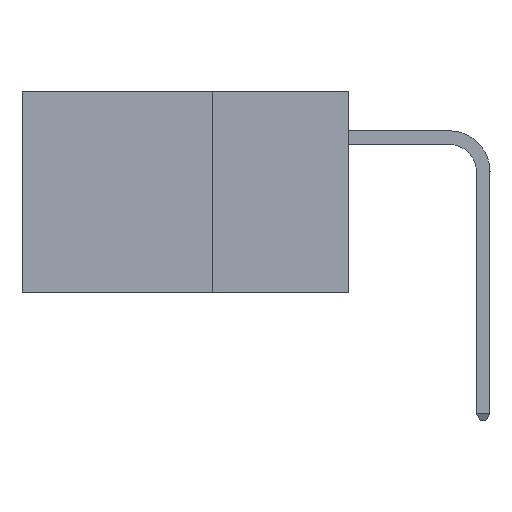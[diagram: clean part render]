
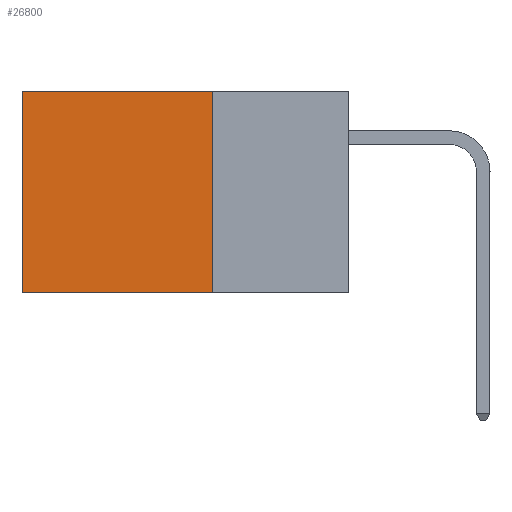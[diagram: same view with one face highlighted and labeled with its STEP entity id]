
A CAD part, left-side view. The second image highlights one B-rep face of the part: STEP entity #26800.
In plain terms, the highlighted planar face has unit normal (-1, 0, 0).
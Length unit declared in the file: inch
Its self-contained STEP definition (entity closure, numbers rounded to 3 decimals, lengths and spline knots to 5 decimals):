
#557 = AXIS2_PLACEMENT_3D ( 'NONE', #37824, #31231, #34038 ) ;
#2293 = VECTOR ( 'NONE', #39726, 39.37008 ) ;
#2990 = DIRECTION ( 'NONE',  ( 0., 1., 0. ) ) ;
#7943 = CARTESIAN_POINT ( 'NONE',  ( 0.2875, 0.25, -0.37 ) ) ;
#8426 = VERTEX_POINT ( 'NONE', #20932 ) ;
#8679 = ORIENTED_EDGE ( 'NONE', *, *, #34176, .F. ) ;
#10671 = LINE ( 'NONE', #29616, #2293 ) ;
#12852 = ORIENTED_EDGE ( 'NONE', *, *, #26646, .T. ) ;
#12959 = CARTESIAN_POINT ( 'NONE',  ( 0.2875, 0.25, -0.37 ) ) ;
#13075 = CARTESIAN_POINT ( 'NONE',  ( 0.2875, 0.6, 0. ) ) ;
#13395 = EDGE_CURVE ( 'NONE', #13584, #17187, #36282, .T. ) ;
#13584 = VERTEX_POINT ( 'NONE', #7943 ) ;
#17187 = VERTEX_POINT ( 'NONE', #40276 ) ;
#18881 = VECTOR ( 'NONE', #23900, 39.37008 ) ;
#19662 = FACE_OUTER_BOUND ( 'NONE', #22738, .T. ) ;
#20932 = CARTESIAN_POINT ( 'NONE',  ( 0.2875, 0.25, 0. ) ) ;
#22738 = EDGE_LOOP ( 'NONE', ( #35744, #42518, #8679, #12852 ) ) ;
#23900 = DIRECTION ( 'NONE',  ( 0., 0., -1. ) ) ;
#24694 = VERTEX_POINT ( 'NONE', #13075 ) ;
#24726 = VECTOR ( 'NONE', #2990, 39.37008 ) ;
#26646 = EDGE_CURVE ( 'NONE', #8426, #24694, #42800, .T. ) ;
#26800 = ADVANCED_FACE ( 'NONE', ( #19662 ), #27573, .F. ) ;
#27573 = PLANE ( 'NONE',  #557 ) ;
#29616 = CARTESIAN_POINT ( 'NONE',  ( 0.2875, 0.6, 0. ) ) ;
#31231 = DIRECTION ( 'NONE',  ( 1., 0., 0. ) ) ;
#34038 = DIRECTION ( 'NONE',  ( 0., 0., -1. ) ) ;
#34176 = EDGE_CURVE ( 'NONE', #8426, #13584, #38304, .T. ) ;
#34338 = CARTESIAN_POINT ( 'NONE',  ( 0.2875, 0.25, 0. ) ) ;
#35744 = ORIENTED_EDGE ( 'NONE', *, *, #41413, .T. ) ;
#36282 = LINE ( 'NONE', #12959, #24726 ) ;
#37824 = CARTESIAN_POINT ( 'NONE',  ( 0.2875, 0.25, 0. ) ) ;
#38304 = LINE ( 'NONE', #34338, #18881 ) ;
#39629 = VECTOR ( 'NONE', #43272, 39.37008 ) ;
#39726 = DIRECTION ( 'NONE',  ( 0., 0., -1. ) ) ;
#40276 = CARTESIAN_POINT ( 'NONE',  ( 0.2875, 0.6, -0.37 ) ) ;
#41413 = EDGE_CURVE ( 'NONE', #24694, #17187, #10671, .T. ) ;
#42518 = ORIENTED_EDGE ( 'NONE', *, *, #13395, .F. ) ;
#42800 = LINE ( 'NONE', #43418, #39629 ) ;
#43272 = DIRECTION ( 'NONE',  ( 0., 1., 0. ) ) ;
#43418 = CARTESIAN_POINT ( 'NONE',  ( 0.2875, 0.25, 0. ) ) ;
